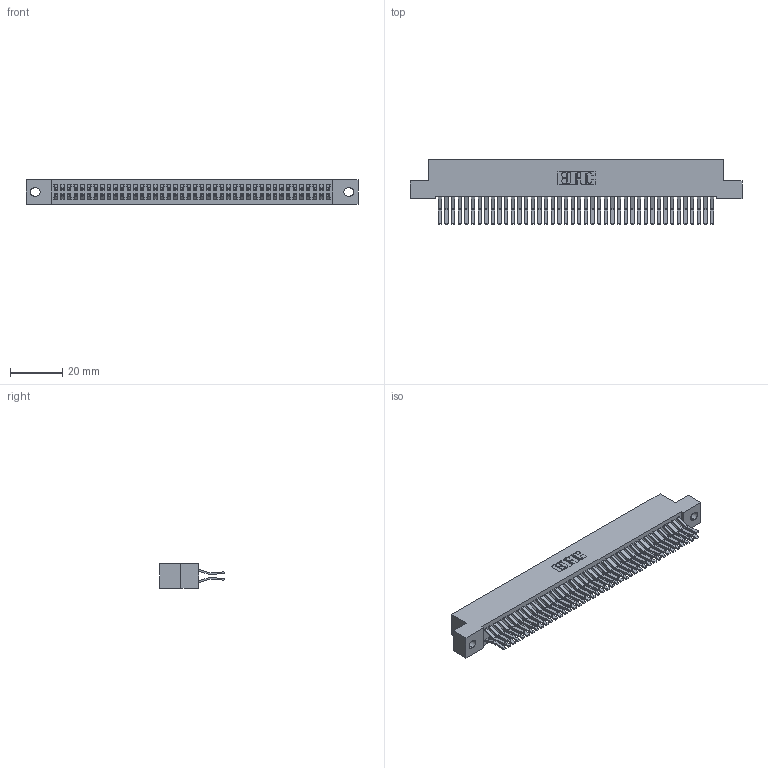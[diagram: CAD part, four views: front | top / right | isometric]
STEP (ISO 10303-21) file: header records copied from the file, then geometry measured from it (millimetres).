
FILE_DESCRIPTION (( 'STEP AP203' ), '1' );
FILE_NAME ('392-084-560-202.STEP', '2018-08-18T04:56:05', ( '' ), ( '' ), 'SwSTEP 2.0', 'SolidWorks 2016', '' );
FILE_SCHEMA (( 'CONFIG_CONTROL_DESIGN' ));
Length unit declared in the file: inch
Products named in the file (3): 342 Part_.128 Slot; 345-292-001_560 Tail; 392-084-560-202
Assembly tree (85 placements, depth 2):
  392-084-560-202
    342 Part_.128 Slot
    345-292-001_560 Tail  x84
Bounding box: 127 x 24.78 x 9.4 mm (x, y, z)
Volume: 11910.3 mm3; surface area: 20468.8 mm2
Topology: 85 solids, 85 shells, 4650 faces, 13835 edges, 9110 vertices
Faces by surface type: plane 3094, cylinder 1556
Entity records: 27111 total; most frequent: CARTESIAN_POINT 4494, ORIENTED_EDGE 4430, DIRECTION 3843, EDGE_CURVE 2215, LINE 2083, VECTOR 2083, VERTEX_POINT 1474, AXIS2_PLACEMENT_3D 880
